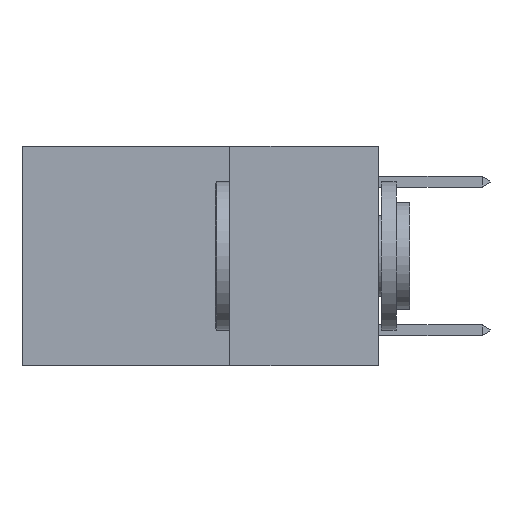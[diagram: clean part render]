
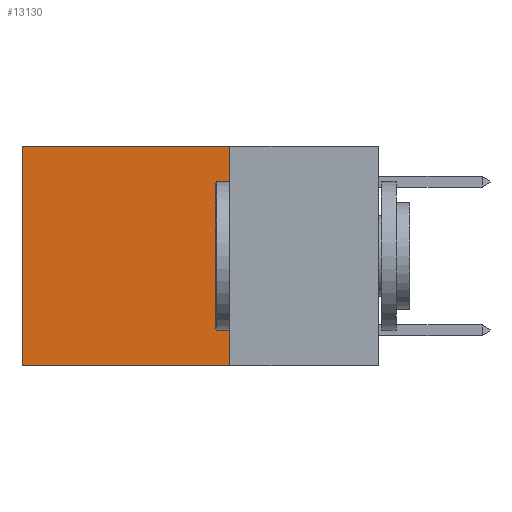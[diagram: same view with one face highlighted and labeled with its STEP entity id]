
A CAD part, left-side view. The second image highlights one B-rep face of the part: STEP entity #13130.
In plain terms, the highlighted planar face has unit normal (-1, 0, 0).
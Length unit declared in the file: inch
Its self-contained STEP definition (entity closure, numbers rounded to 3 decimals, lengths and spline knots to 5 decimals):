
#67 = VECTOR ( 'NONE', #10470, 39.37008 ) ;
#824 = ORIENTED_EDGE ( 'NONE', *, *, #11973, .T. ) ;
#2006 = DIRECTION ( 'NONE',  ( 1., 0., 0. ) ) ;
#2113 = ORIENTED_EDGE ( 'NONE', *, *, #6637, .T. ) ;
#2906 = CARTESIAN_POINT ( 'NONE',  ( 0.2625, 0.25, -0.37 ) ) ;
#3725 = EDGE_CURVE ( 'NONE', #10973, #5584, #8722, .T. ) ;
#3991 = LINE ( 'NONE', #8668, #10579 ) ;
#4048 = ORIENTED_EDGE ( 'NONE', *, *, #3725, .F. ) ;
#4340 = LINE ( 'NONE', #8861, #5507 ) ;
#4863 = VECTOR ( 'NONE', #9028, 39.37008 ) ;
#5507 = VECTOR ( 'NONE', #6499, 39.37008 ) ;
#5584 = VERTEX_POINT ( 'NONE', #14852 ) ;
#5728 = EDGE_LOOP ( 'NONE', ( #824, #4048, #6799, #2113 ) ) ;
#5775 = LINE ( 'NONE', #6691, #67 ) ;
#6499 = DIRECTION ( 'NONE',  ( 0., 0., -1. ) ) ;
#6637 = EDGE_CURVE ( 'NONE', #13906, #9485, #3991, .T. ) ;
#6691 = CARTESIAN_POINT ( 'NONE',  ( 0.2625, 0.25, 0. ) ) ;
#6748 = AXIS2_PLACEMENT_3D ( 'NONE', #7831, #2006, #10209 ) ;
#6799 = ORIENTED_EDGE ( 'NONE', *, *, #7606, .F. ) ;
#7606 = EDGE_CURVE ( 'NONE', #13906, #10973, #5775, .T. ) ;
#7831 = CARTESIAN_POINT ( 'NONE',  ( 0.2625, 0.25, 0. ) ) ;
#8668 = CARTESIAN_POINT ( 'NONE',  ( 0.2625, 0.25, 0. ) ) ;
#8722 = LINE ( 'NONE', #2906, #4863 ) ;
#8748 = DIRECTION ( 'NONE',  ( 0., 1., 0. ) ) ;
#8861 = CARTESIAN_POINT ( 'NONE',  ( 0.2625, 0.6, 0. ) ) ;
#9028 = DIRECTION ( 'NONE',  ( 0., 1., 0. ) ) ;
#9485 = VERTEX_POINT ( 'NONE', #12975 ) ;
#10209 = DIRECTION ( 'NONE',  ( 0., 0., -1. ) ) ;
#10470 = DIRECTION ( 'NONE',  ( 0., 0., -1. ) ) ;
#10579 = VECTOR ( 'NONE', #8748, 39.37008 ) ;
#10924 = CARTESIAN_POINT ( 'NONE',  ( 0.2625, 0.25, -0.37 ) ) ;
#10973 = VERTEX_POINT ( 'NONE', #10924 ) ;
#11355 = FACE_OUTER_BOUND ( 'NONE', #5728, .T. ) ;
#11973 = EDGE_CURVE ( 'NONE', #9485, #5584, #4340, .T. ) ;
#12462 = CARTESIAN_POINT ( 'NONE',  ( 0.2625, 0.25, 0. ) ) ;
#12975 = CARTESIAN_POINT ( 'NONE',  ( 0.2625, 0.6, 0. ) ) ;
#13130 = ADVANCED_FACE ( 'NONE', ( #11355 ), #15042, .F. ) ;
#13906 = VERTEX_POINT ( 'NONE', #12462 ) ;
#14852 = CARTESIAN_POINT ( 'NONE',  ( 0.2625, 0.6, -0.37 ) ) ;
#15042 = PLANE ( 'NONE',  #6748 ) ;
